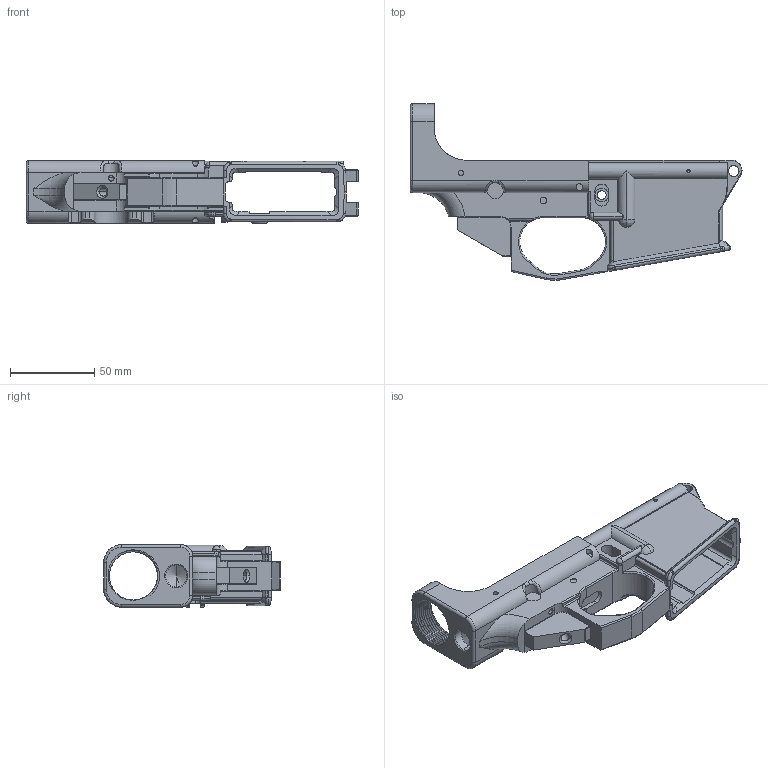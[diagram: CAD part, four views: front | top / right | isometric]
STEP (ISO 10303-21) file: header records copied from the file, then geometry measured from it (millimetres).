
FILE_DESCRIPTION((''),'2;1');
FILE_NAME('DEFDIST_','2013-04-06T',('fireraisr'),(''),'PRO/ENGINEER BY PARAMETRIC TECHNOLOGY CORPORATION, 2007450','PRO/ENGINEER BY PARAMETRIC TECHNOLOGY CORPORATION, 2007450','');
FILE_SCHEMA(('CONFIG_CONTROL_DESIGN'));
Length unit declared in the file: inch
Products named in the file (1): DEFDIST_
Bounding box: 197.08 x 104.92 x 37.19 mm (x, y, z)
Volume: 163532.2 mm3; surface area: 57357.4 mm2
Topology: 1 solids, 2 shells, 906 faces, 2460 edges, 1583 vertices
Faces by surface type: plane 417, cylinder 263, extrusion 92, bspline 64, torus 51, cone 12, sphere 7
Entity records: 39251 total; most frequent: CARTESIAN_POINT 17431, ORIENTED_EDGE 4894, DIRECTION 3877, EDGE_CURVE 2447, VERTEX_POINT 1583, VECTOR 1511, LINE 1419, AXIS2_PLACEMENT_3D 1183
